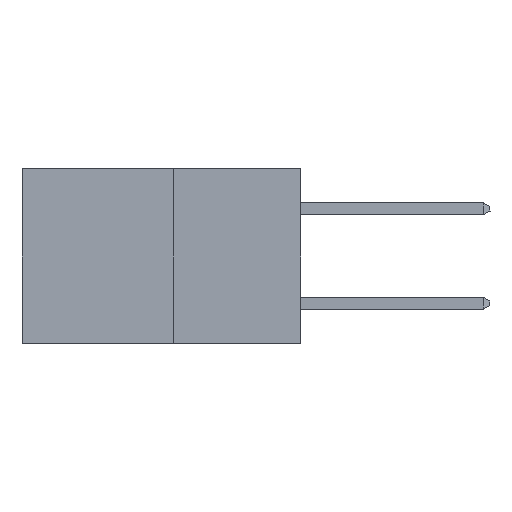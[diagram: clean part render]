
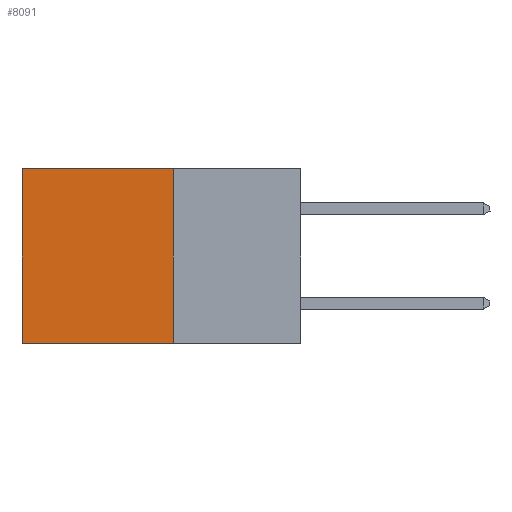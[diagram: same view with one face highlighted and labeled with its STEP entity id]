
A CAD part, left-side view. The second image highlights one B-rep face of the part: STEP entity #8091.
In plain terms, the highlighted planar face has unit normal (-1, 0, 0).
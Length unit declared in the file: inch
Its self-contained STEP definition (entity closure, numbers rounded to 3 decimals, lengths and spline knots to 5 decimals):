
#1626 = EDGE_CURVE ( 'NONE', #24759, #6802, #24487, .T. ) ;
#2405 = DIRECTION ( 'NONE',  ( 0., 0., -1. ) ) ;
#2529 = DIRECTION ( 'NONE',  ( 0., 1., 0. ) ) ;
#2711 = DIRECTION ( 'NONE',  ( 0., 0., -1. ) ) ;
#2769 = CARTESIAN_POINT ( 'NONE',  ( 0.277, 0.59, 0. ) ) ;
#4394 = CARTESIAN_POINT ( 'NONE',  ( 0.277, 0.27, 0. ) ) ;
#4571 = PLANE ( 'NONE',  #13958 ) ;
#5494 = ORIENTED_EDGE ( 'NONE', *, *, #10972, .T. ) ;
#5700 = CARTESIAN_POINT ( 'NONE',  ( 0.277, 0.27, -0.37 ) ) ;
#6353 = DIRECTION ( 'NONE',  ( 0., 0., -1. ) ) ;
#6802 = VERTEX_POINT ( 'NONE', #2769 ) ;
#6877 = CARTESIAN_POINT ( 'NONE',  ( 0.277, 0.27, -0.37 ) ) ;
#6981 = VECTOR ( 'NONE', #23278, 39.37008 ) ;
#8091 = ADVANCED_FACE ( 'NONE', ( #15885 ), #4571, .F. ) ;
#8315 = ORIENTED_EDGE ( 'NONE', *, *, #1626, .T. ) ;
#8476 = EDGE_LOOP ( 'NONE', ( #5494, #8835, #19090, #8315 ) ) ;
#8580 = CARTESIAN_POINT ( 'NONE',  ( 0.277, 0.59, -0.37 ) ) ;
#8835 = ORIENTED_EDGE ( 'NONE', *, *, #17462, .F. ) ;
#10972 = EDGE_CURVE ( 'NONE', #6802, #25731, #14717, .T. ) ;
#11161 = CARTESIAN_POINT ( 'NONE',  ( 0.277, 0.59, -0.37 ) ) ;
#13734 = CARTESIAN_POINT ( 'NONE',  ( 0.277, 0.27, -0.37 ) ) ;
#13958 = AXIS2_PLACEMENT_3D ( 'NONE', #26607, #15597, #2405 ) ;
#14717 = LINE ( 'NONE', #8580, #19211 ) ;
#15597 = DIRECTION ( 'NONE',  ( 1., 0., 0. ) ) ;
#15885 = FACE_OUTER_BOUND ( 'NONE', #8476, .T. ) ;
#16517 = LINE ( 'NONE', #13734, #21661 ) ;
#17240 = VECTOR ( 'NONE', #2529, 39.37008 ) ;
#17462 = EDGE_CURVE ( 'NONE', #22086, #25731, #17947, .T. ) ;
#17947 = LINE ( 'NONE', #5700, #6981 ) ;
#18859 = EDGE_CURVE ( 'NONE', #24759, #22086, #16517, .T. ) ;
#19090 = ORIENTED_EDGE ( 'NONE', *, *, #18859, .F. ) ;
#19211 = VECTOR ( 'NONE', #6353, 39.37008 ) ;
#21661 = VECTOR ( 'NONE', #2711, 39.37008 ) ;
#22086 = VERTEX_POINT ( 'NONE', #6877 ) ;
#23278 = DIRECTION ( 'NONE',  ( 0., 1., 0. ) ) ;
#24487 = LINE ( 'NONE', #4394, #17240 ) ;
#24759 = VERTEX_POINT ( 'NONE', #25744 ) ;
#25731 = VERTEX_POINT ( 'NONE', #11161 ) ;
#25744 = CARTESIAN_POINT ( 'NONE',  ( 0.277, 0.27, 0. ) ) ;
#26607 = CARTESIAN_POINT ( 'NONE',  ( 0.277, 0.27, -0.37 ) ) ;
